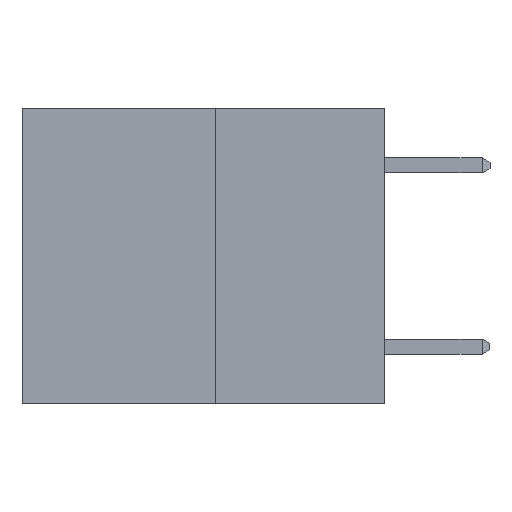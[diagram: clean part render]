
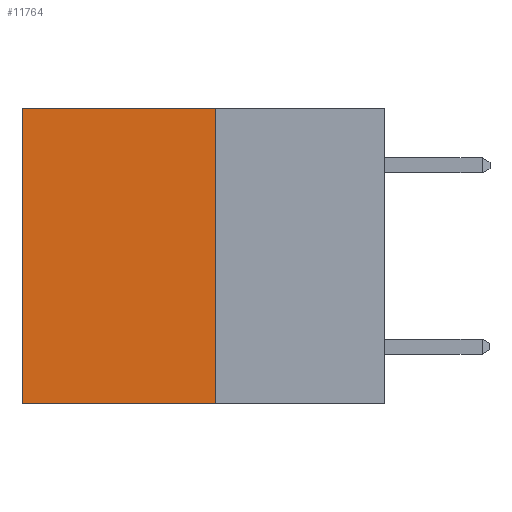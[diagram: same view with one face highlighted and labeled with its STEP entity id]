
A CAD part, left-side view. The second image highlights one B-rep face of the part: STEP entity #11764.
In plain terms, the highlighted planar face has unit normal (-1, 0, 0).
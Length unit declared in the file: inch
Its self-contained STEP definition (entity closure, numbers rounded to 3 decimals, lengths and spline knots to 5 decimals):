
#316 = LINE ( 'NONE', #8824, #13046 ) ;
#1266 = VECTOR ( 'NONE', #5454, 39.37008 ) ;
#1273 = DIRECTION ( 'NONE',  ( 0., 0., -1. ) ) ;
#1410 = CARTESIAN_POINT ( 'NONE',  ( 0.3165, 0.28, 0. ) ) ;
#1626 = VECTOR ( 'NONE', #7625, 39.37008 ) ;
#2129 = AXIS2_PLACEMENT_3D ( 'NONE', #6683, #6724, #1273 ) ;
#2450 = FACE_OUTER_BOUND ( 'NONE', #8120, .T. ) ;
#2978 = CARTESIAN_POINT ( 'NONE',  ( 0.3165, 0.6, -0.49 ) ) ;
#3832 = LINE ( 'NONE', #11014, #1266 ) ;
#4949 = ORIENTED_EDGE ( 'NONE', *, *, #12269, .T. ) ;
#5454 = DIRECTION ( 'NONE',  ( 0., 0., -1. ) ) ;
#5485 = CARTESIAN_POINT ( 'NONE',  ( 0.3165, 0.28, -0.49 ) ) ;
#5834 = DIRECTION ( 'NONE',  ( 0., 1., 0. ) ) ;
#5917 = VERTEX_POINT ( 'NONE', #1410 ) ;
#6646 = EDGE_CURVE ( 'NONE', #11485, #8325, #316, .T. ) ;
#6683 = CARTESIAN_POINT ( 'NONE',  ( 0.3165, 0.28, -0.49 ) ) ;
#6724 = DIRECTION ( 'NONE',  ( 1., 0., 0. ) ) ;
#7625 = DIRECTION ( 'NONE',  ( 0., 0., -1. ) ) ;
#7821 = ORIENTED_EDGE ( 'NONE', *, *, #14036, .F. ) ;
#8067 = CARTESIAN_POINT ( 'NONE',  ( 0.3165, 0.28, 0. ) ) ;
#8120 = EDGE_LOOP ( 'NONE', ( #4949, #10235, #7821, #9442 ) ) ;
#8325 = VERTEX_POINT ( 'NONE', #2978 ) ;
#8824 = CARTESIAN_POINT ( 'NONE',  ( 0.3165, 0.28, -0.49 ) ) ;
#8921 = PLANE ( 'NONE',  #2129 ) ;
#9116 = CARTESIAN_POINT ( 'NONE',  ( 0.3165, 0.6, 0. ) ) ;
#9442 = ORIENTED_EDGE ( 'NONE', *, *, #10522, .T. ) ;
#9704 = VERTEX_POINT ( 'NONE', #9116 ) ;
#9715 = VECTOR ( 'NONE', #5834, 39.37008 ) ;
#10235 = ORIENTED_EDGE ( 'NONE', *, *, #6646, .F. ) ;
#10522 = EDGE_CURVE ( 'NONE', #5917, #9704, #14152, .T. ) ;
#10752 = LINE ( 'NONE', #5485, #1626 ) ;
#11014 = CARTESIAN_POINT ( 'NONE',  ( 0.3165, 0.6, -0.49 ) ) ;
#11485 = VERTEX_POINT ( 'NONE', #11742 ) ;
#11742 = CARTESIAN_POINT ( 'NONE',  ( 0.3165, 0.28, -0.49 ) ) ;
#11764 = ADVANCED_FACE ( 'NONE', ( #2450 ), #8921, .F. ) ;
#12269 = EDGE_CURVE ( 'NONE', #9704, #8325, #3832, .T. ) ;
#13046 = VECTOR ( 'NONE', #14168, 39.37008 ) ;
#14036 = EDGE_CURVE ( 'NONE', #5917, #11485, #10752, .T. ) ;
#14152 = LINE ( 'NONE', #8067, #9715 ) ;
#14168 = DIRECTION ( 'NONE',  ( 0., 1., 0. ) ) ;
